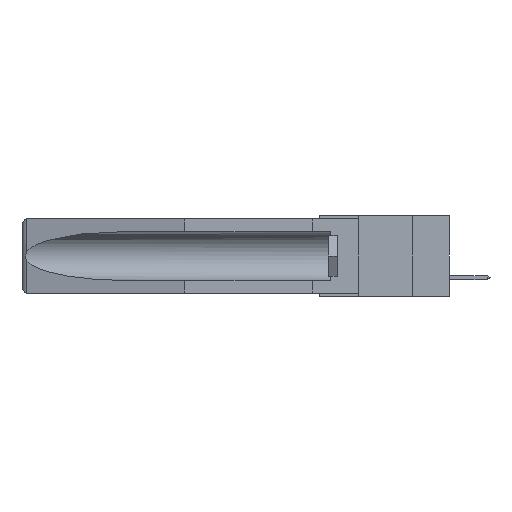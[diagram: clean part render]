
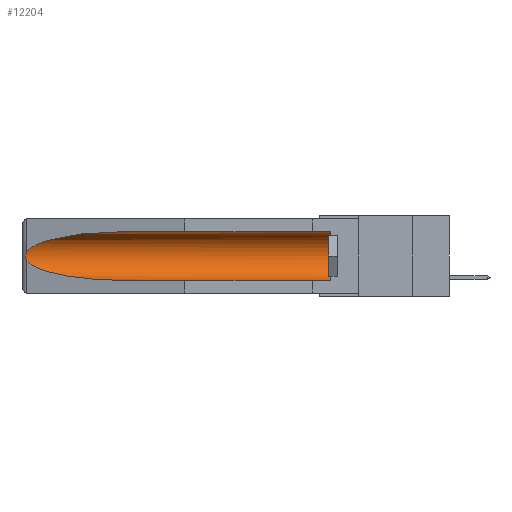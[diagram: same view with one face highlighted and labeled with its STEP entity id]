
A CAD part, left-side view. The second image highlights one B-rep face of the part: STEP entity #12204.
In plain terms, the highlighted cylindrical face has radius 2.857 mm (diameter 5.715 mm), a partial arc.
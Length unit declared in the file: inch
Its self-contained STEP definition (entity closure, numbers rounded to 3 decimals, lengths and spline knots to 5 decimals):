
#186 = CARTESIAN_POINT ( 'NONE',  ( 0.155, 1.07973, -0.059 ) ) ;
#337 = LINE ( 'NONE', #15752, #17456 ) ;
#737 = LINE ( 'NONE', #8947, #29528 ) ;
#1512 = ORIENTED_EDGE ( 'NONE', *, *, #2104, .T. ) ;
#1565 = CARTESIAN_POINT ( 'NONE',  ( 0.26597, 1.52961, -0.15275 ) ) ;
#1783 = CARTESIAN_POINT ( 'NONE',  ( 0.26537, 1.52718, -0.14972 ) ) ;
#2104 = EDGE_CURVE ( 'NONE', #24953, #21141, #5760, .T. ) ;
#2148 = CIRCLE ( 'NONE', #20200, 0.1125 ) ;
#2933 = CARTESIAN_POINT ( 'NONE',  ( 0.26537, 1.52718, -0.19328 ) ) ;
#4017 = CARTESIAN_POINT ( 'NONE',  ( 0.26537, 1.52718, -0.19328 ) ) ;
#5229 =( BOUNDED_CURVE ( )  B_SPLINE_CURVE ( 3, ( #2933, #12983, #12785, #29287 ),
 .UNSPECIFIED., .F., .F. ) 
 B_SPLINE_CURVE_WITH_KNOTS ( ( 4, 4 ),
 ( 0.1948, 1.5708 ),
 .UNSPECIFIED. ) 
 CURVE ( )  GEOMETRIC_REPRESENTATION_ITEM ( )  RATIONAL_B_SPLINE_CURVE ( ( 1., 0.848, 0.848, 1. ) ) 
 REPRESENTATION_ITEM ( '' )  );
#5339 = CARTESIAN_POINT ( 'NONE',  ( 0.155, 0.126, -0.284 ) ) ;
#5760 =( BOUNDED_CURVE ( )  B_SPLINE_CURVE ( 3, ( #7889, #28874, #23345, #11736 ),
 .UNSPECIFIED., .F., .F. ) 
 B_SPLINE_CURVE_WITH_KNOTS ( ( 4, 4 ),
 ( 4.71239, 6.08839 ),
 .UNSPECIFIED. ) 
 CURVE ( )  GEOMETRIC_REPRESENTATION_ITEM ( )  RATIONAL_B_SPLINE_CURVE ( ( 1., 0.848, 0.848, 1. ) ) 
 REPRESENTATION_ITEM ( '' )  );
#6105 = VERTEX_POINT ( 'NONE', #19646 ) ;
#6724 = CARTESIAN_POINT ( 'NONE',  ( 0.26537, 1.52718, -0.19328 ) ) ;
#7889 = CARTESIAN_POINT ( 'NONE',  ( 0.155, 1.07973, -0.059 ) ) ;
#8177 = EDGE_CURVE ( 'NONE', #8750, #6105, #5229, .T. ) ;
#8678 = CARTESIAN_POINT ( 'NONE',  ( 0.2673, 1.5327, -0.16383 ) ) ;
#8750 = VERTEX_POINT ( 'NONE', #6724 ) ;
#8947 = CARTESIAN_POINT ( 'NONE',  ( 0.155, -0.30754, -0.059 ) ) ;
#9675 = VERTEX_POINT ( 'NONE', #5339 ) ;
#9980 = FACE_OUTER_BOUND ( 'NONE', #14638, .T. ) ;
#11736 = CARTESIAN_POINT ( 'NONE',  ( 0.26537, 1.52718, -0.14972 ) ) ;
#12204 = ADVANCED_FACE ( 'NONE', ( #9980 ), #19422, .F. ) ;
#12785 = CARTESIAN_POINT ( 'NONE',  ( 0.21114, 1.30732, -0.284 ) ) ;
#12983 = CARTESIAN_POINT ( 'NONE',  ( 0.25451, 1.48313, -0.24835 ) ) ;
#14273 = EDGE_CURVE ( 'NONE', #25595, #24953, #737, .T. ) ;
#14638 = EDGE_LOOP ( 'NONE', ( #1512, #30154, #28030, #16588, #25012, #27380 ) ) ;
#15516 = CARTESIAN_POINT ( 'NONE',  ( 0.2675, 1.53308, -0.17534 ) ) ;
#15652 = EDGE_CURVE ( 'NONE', #9675, #25595, #2148, .T. ) ;
#15683 = CARTESIAN_POINT ( 'NONE',  ( 0.155, -0.30754, -0.1715 ) ) ;
#15752 = CARTESIAN_POINT ( 'NONE',  ( 0.155, -0.30754, -0.284 ) ) ;
#16588 = ORIENTED_EDGE ( 'NONE', *, *, #18514, .F. ) ;
#16958 = CARTESIAN_POINT ( 'NONE',  ( 0.26537, 1.52718, -0.14972 ) ) ;
#16973 = EDGE_CURVE ( 'NONE', #21141, #8750, #20701, .T. ) ;
#17456 = VECTOR ( 'NONE', #25094, 39.37008 ) ;
#17851 = CARTESIAN_POINT ( 'NONE',  ( 0.26654, 1.53092, -0.15636 ) ) ;
#18046 = CARTESIAN_POINT ( 'NONE',  ( 0.26655, 1.53094, -0.18657 ) ) ;
#18095 = CARTESIAN_POINT ( 'NONE',  ( 0.155, 0.126, -0.1715 ) ) ;
#18514 = EDGE_CURVE ( 'NONE', #9675, #6105, #337, .T. ) ;
#18599 = DIRECTION ( 'NONE',  ( 0., 1., 0. ) ) ;
#19422 = CYLINDRICAL_SURFACE ( 'NONE', #25720, 0.1125 ) ;
#19646 = CARTESIAN_POINT ( 'NONE',  ( 0.155, 1.07973, -0.284 ) ) ;
#20200 = AXIS2_PLACEMENT_3D ( 'NONE', #18095, #27382, #22668 ) ;
#20701 = B_SPLINE_CURVE_WITH_KNOTS ( 'NONE', 3,
 ( #1783, #1565, #17851, #8678, #22834, #15516, #27444, #18046, #22513, #4017 ),
 .UNSPECIFIED., .F., .F.,
 ( 4, 2, 2, 2, 4 ),
 ( 0., 0.00029, 0.00058, 0.00087, 0.00117 ),
 .UNSPECIFIED. ) ;
#21141 = VERTEX_POINT ( 'NONE', #16958 ) ;
#22177 = DIRECTION ( 'NONE',  ( 0., 0., 1. ) ) ;
#22513 = CARTESIAN_POINT ( 'NONE',  ( 0.26597, 1.5296, -0.19026 ) ) ;
#22668 = DIRECTION ( 'NONE',  ( 0., 0., 1. ) ) ;
#22834 = CARTESIAN_POINT ( 'NONE',  ( 0.2675, 1.53308, -0.16763 ) ) ;
#23345 = CARTESIAN_POINT ( 'NONE',  ( 0.25451, 1.48313, -0.09465 ) ) ;
#24048 = CARTESIAN_POINT ( 'NONE',  ( 0.155, 0.126, -0.059 ) ) ;
#24953 = VERTEX_POINT ( 'NONE', #186 ) ;
#25012 = ORIENTED_EDGE ( 'NONE', *, *, #15652, .T. ) ;
#25094 = DIRECTION ( 'NONE',  ( 0., 1., 0. ) ) ;
#25595 = VERTEX_POINT ( 'NONE', #24048 ) ;
#25720 = AXIS2_PLACEMENT_3D ( 'NONE', #15683, #26985, #22177 ) ;
#26985 = DIRECTION ( 'NONE',  ( 0., 1., 0. ) ) ;
#27380 = ORIENTED_EDGE ( 'NONE', *, *, #14273, .T. ) ;
#27382 = DIRECTION ( 'NONE',  ( 0., -1., 0. ) ) ;
#27444 = CARTESIAN_POINT ( 'NONE',  ( 0.2673, 1.53269, -0.17917 ) ) ;
#28030 = ORIENTED_EDGE ( 'NONE', *, *, #8177, .T. ) ;
#28874 = CARTESIAN_POINT ( 'NONE',  ( 0.21114, 1.30732, -0.059 ) ) ;
#29287 = CARTESIAN_POINT ( 'NONE',  ( 0.155, 1.07973, -0.284 ) ) ;
#29528 = VECTOR ( 'NONE', #18599, 39.37008 ) ;
#30154 = ORIENTED_EDGE ( 'NONE', *, *, #16973, .T. ) ;
